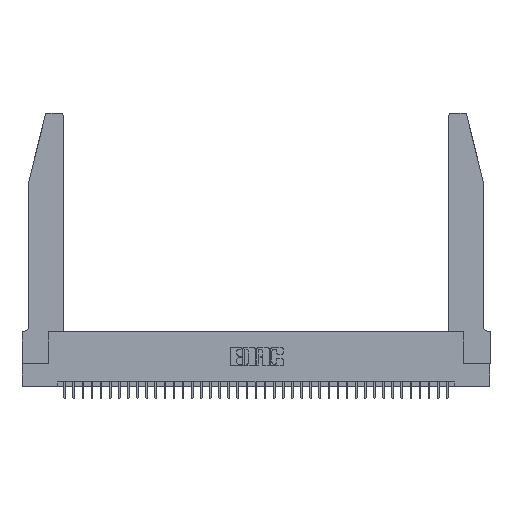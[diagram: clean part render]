
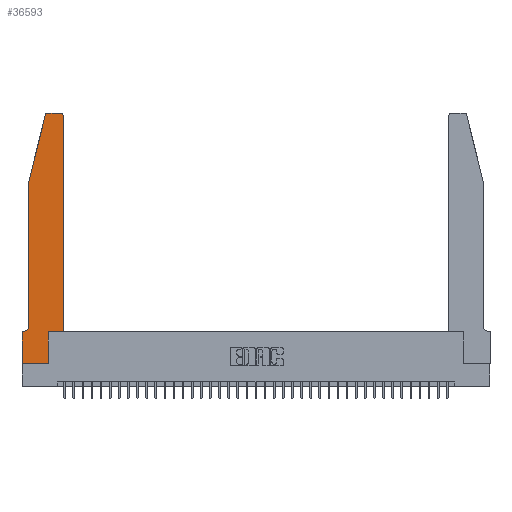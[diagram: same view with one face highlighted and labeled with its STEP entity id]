
A CAD part, top view. The second image highlights one B-rep face of the part: STEP entity #36593.
In plain terms, the highlighted planar face has unit normal (0, 0, 1).
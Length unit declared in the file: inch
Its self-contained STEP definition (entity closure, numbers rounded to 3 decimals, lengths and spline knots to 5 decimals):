
#808 = VERTEX_POINT ( 'NONE', #37695 ) ;
#1588 = ORIENTED_EDGE ( 'NONE', *, *, #15135, .T. ) ;
#2073 = DIRECTION ( 'NONE',  ( 1., 0., 0. ) ) ;
#2214 = EDGE_CURVE ( 'NONE', #3378, #24615, #37303, .T. ) ;
#3378 = VERTEX_POINT ( 'NONE', #8106 ) ;
#3709 = CARTESIAN_POINT ( 'NONE',  ( 0.2865, 0., 0.37 ) ) ;
#3925 = EDGE_CURVE ( 'NONE', #30119, #35754, #37261, .T. ) ;
#4754 = LINE ( 'NONE', #25187, #28563 ) ;
#4790 = CARTESIAN_POINT ( 'NONE',  ( 0.0755, 2., 0.37 ) ) ;
#4828 = CARTESIAN_POINT ( 'NONE',  ( 0.0755, 2., 0.37 ) ) ;
#5068 = EDGE_LOOP ( 'NONE', ( #15764, #7816, #27701, #36129, #15210, #17078, #15665, #38114, #28882, #17957, #6788, #1588 ) ) ;
#5127 = CARTESIAN_POINT ( 'NONE',  ( 0.2865, 0.35, 0.37 ) ) ;
#5841 = LINE ( 'NONE', #23164, #17727 ) ;
#6004 = VECTOR ( 'NONE', #23053, 39.37008 ) ;
#6175 = CARTESIAN_POINT ( 'NONE',  ( 0.4505, 0.35, 0.37 ) ) ;
#6788 = ORIENTED_EDGE ( 'NONE', *, *, #17180, .T. ) ;
#7801 = CARTESIAN_POINT ( 'NONE',  ( 0.0055, 0.42, 0.37 ) ) ;
#7816 = ORIENTED_EDGE ( 'NONE', *, *, #22399, .T. ) ;
#8106 = CARTESIAN_POINT ( 'NONE',  ( 0.0755, 2., 0.37 ) ) ;
#8332 = EDGE_CURVE ( 'NONE', #16528, #35789, #31956, .T. ) ;
#8527 = AXIS2_PLACEMENT_3D ( 'NONE', #23153, #37219, #16952 ) ;
#8632 = CARTESIAN_POINT ( 'NONE',  ( 0.284, 2.75, 0.37 ) ) ;
#11556 = DIRECTION ( 'NONE',  ( 1., 0., 0. ) ) ;
#11580 = CARTESIAN_POINT ( 'NONE',  ( 0., 0.35, 0.37 ) ) ;
#13168 = DIRECTION ( 'NONE',  ( 0., 0., 1. ) ) ;
#13833 = CARTESIAN_POINT ( 'NONE',  ( 0.4505, 0.35, 0.37 ) ) ;
#13847 = PLANE ( 'NONE',  #8527 ) ;
#14233 = FACE_OUTER_BOUND ( 'NONE', #5068, .T. ) ;
#14519 = LINE ( 'NONE', #20543, #17863 ) ;
#14778 = EDGE_CURVE ( 'NONE', #35754, #21761, #14519, .T. ) ;
#15135 = EDGE_CURVE ( 'NONE', #808, #33713, #20377, .T. ) ;
#15210 = ORIENTED_EDGE ( 'NONE', *, *, #17246, .T. ) ;
#15375 = AXIS2_PLACEMENT_3D ( 'NONE', #36330, #13168, #25210 ) ;
#15665 = ORIENTED_EDGE ( 'NONE', *, *, #26588, .T. ) ;
#15764 = ORIENTED_EDGE ( 'NONE', *, *, #19226, .T. ) ;
#16441 = DIRECTION ( 'NONE',  ( 0., -1., 0. ) ) ;
#16482 = LINE ( 'NONE', #28337, #37606 ) ;
#16528 = VERTEX_POINT ( 'NONE', #36278 ) ;
#16705 = DIRECTION ( 'NONE',  ( -0.239, -0.971, 0. ) ) ;
#16752 = DIRECTION ( 'NONE',  ( -1., 0., 0. ) ) ;
#16836 = CARTESIAN_POINT ( 'NONE',  ( 0.4205, 2.72, 0.37 ) ) ;
#16952 = DIRECTION ( 'NONE',  ( 1., 0., 0. ) ) ;
#17041 = CARTESIAN_POINT ( 'NONE',  ( 0.2865, 0.35, 0.37 ) ) ;
#17078 = ORIENTED_EDGE ( 'NONE', *, *, #8332, .T. ) ;
#17180 = EDGE_CURVE ( 'NONE', #21761, #808, #34853, .T. ) ;
#17246 = EDGE_CURVE ( 'NONE', #24615, #16528, #34989, .T. ) ;
#17727 = VECTOR ( 'NONE', #37790, 39.37008 ) ;
#17735 = CARTESIAN_POINT ( 'NONE',  ( 0.0755, 0.35, 0.37 ) ) ;
#17863 = VECTOR ( 'NONE', #2073, 39.37008 ) ;
#17957 = ORIENTED_EDGE ( 'NONE', *, *, #14778, .T. ) ;
#19226 = EDGE_CURVE ( 'NONE', #33713, #21165, #16482, .T. ) ;
#20181 = EDGE_CURVE ( 'NONE', #29161, #30119, #5841, .T. ) ;
#20377 = CIRCLE ( 'NONE', #34686, 0.03 ) ;
#20421 = DIRECTION ( 'NONE',  ( 0., 0., -1. ) ) ;
#20543 = CARTESIAN_POINT ( 'NONE',  ( 0.4505, 0.35, 0.37 ) ) ;
#20907 = VECTOR ( 'NONE', #16705, 39.37008 ) ;
#21165 = VERTEX_POINT ( 'NONE', #8632 ) ;
#21761 = VERTEX_POINT ( 'NONE', #6175 ) ;
#22399 = EDGE_CURVE ( 'NONE', #21165, #22595, #34645, .T. ) ;
#22482 = CARTESIAN_POINT ( 'NONE',  ( 0.25487, 2.72718, 0.37 ) ) ;
#22573 = AXIS2_PLACEMENT_3D ( 'NONE', #7801, #20421, #16752 ) ;
#22595 = VERTEX_POINT ( 'NONE', #22482 ) ;
#23053 = DIRECTION ( 'NONE',  ( 0., -1., 0. ) ) ;
#23153 = CARTESIAN_POINT ( 'NONE',  ( 0., 0.35, 0.37 ) ) ;
#23164 = CARTESIAN_POINT ( 'NONE',  ( 0., 0., 0.37 ) ) ;
#23261 = EDGE_CURVE ( 'NONE', #22595, #3378, #28177, .T. ) ;
#24615 = VERTEX_POINT ( 'NONE', #38083 ) ;
#24698 = CARTESIAN_POINT ( 'NONE',  ( 0.4205, 2.75, 0.37 ) ) ;
#25187 = CARTESIAN_POINT ( 'NONE',  ( 0., 0., 0.37 ) ) ;
#25210 = DIRECTION ( 'NONE',  ( 1., 0., 0. ) ) ;
#26588 = EDGE_CURVE ( 'NONE', #35789, #29161, #4754, .T. ) ;
#27701 = ORIENTED_EDGE ( 'NONE', *, *, #23261, .T. ) ;
#28177 = LINE ( 'NONE', #4828, #20907 ) ;
#28337 = CARTESIAN_POINT ( 'NONE',  ( 0.2605, 2.75, 0.37 ) ) ;
#28563 = VECTOR ( 'NONE', #16441, 39.37008 ) ;
#28882 = ORIENTED_EDGE ( 'NONE', *, *, #3925, .T. ) ;
#29161 = VERTEX_POINT ( 'NONE', #31724 ) ;
#29983 = VECTOR ( 'NONE', #38359, 39.37008 ) ;
#30119 = VERTEX_POINT ( 'NONE', #3709 ) ;
#31724 = CARTESIAN_POINT ( 'NONE',  ( 0., 0., 0.37 ) ) ;
#31916 = DIRECTION ( 'NONE',  ( 0., 1., 0. ) ) ;
#31956 = LINE ( 'NONE', #17735, #29983 ) ;
#31998 = DIRECTION ( 'NONE',  ( 0., 0., 1. ) ) ;
#33713 = VERTEX_POINT ( 'NONE', #24698 ) ;
#33880 = VECTOR ( 'NONE', #37072, 39.37008 ) ;
#34645 = CIRCLE ( 'NONE', #15375, 0.03 ) ;
#34686 = AXIS2_PLACEMENT_3D ( 'NONE', #16836, #31998, #11556 ) ;
#34853 = LINE ( 'NONE', #13833, #36895 ) ;
#34989 = CIRCLE ( 'NONE', #22573, 0.07 ) ;
#35754 = VERTEX_POINT ( 'NONE', #17041 ) ;
#35789 = VERTEX_POINT ( 'NONE', #11580 ) ;
#36129 = ORIENTED_EDGE ( 'NONE', *, *, #2214, .T. ) ;
#36278 = CARTESIAN_POINT ( 'NONE',  ( 0.0055, 0.35, 0.37 ) ) ;
#36330 = CARTESIAN_POINT ( 'NONE',  ( 0.284, 2.72, 0.37 ) ) ;
#36593 = ADVANCED_FACE ( 'NONE', ( #14233 ), #13847, .T. ) ;
#36895 = VECTOR ( 'NONE', #31916, 39.37008 ) ;
#37072 = DIRECTION ( 'NONE',  ( 0., 1., 0. ) ) ;
#37219 = DIRECTION ( 'NONE',  ( 0., 0., 1. ) ) ;
#37261 = LINE ( 'NONE', #5127, #33880 ) ;
#37303 = LINE ( 'NONE', #4790, #6004 ) ;
#37314 = DIRECTION ( 'NONE',  ( -1., 0., 0. ) ) ;
#37606 = VECTOR ( 'NONE', #37314, 39.37008 ) ;
#37695 = CARTESIAN_POINT ( 'NONE',  ( 0.4505, 2.72, 0.37 ) ) ;
#37790 = DIRECTION ( 'NONE',  ( 1., 0., 0. ) ) ;
#38083 = CARTESIAN_POINT ( 'NONE',  ( 0.0755, 0.42, 0.37 ) ) ;
#38114 = ORIENTED_EDGE ( 'NONE', *, *, #20181, .T. ) ;
#38359 = DIRECTION ( 'NONE',  ( -1., 0., 0. ) ) ;
